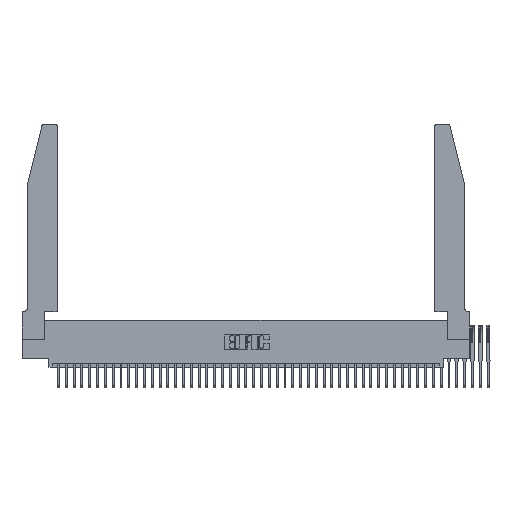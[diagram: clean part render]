
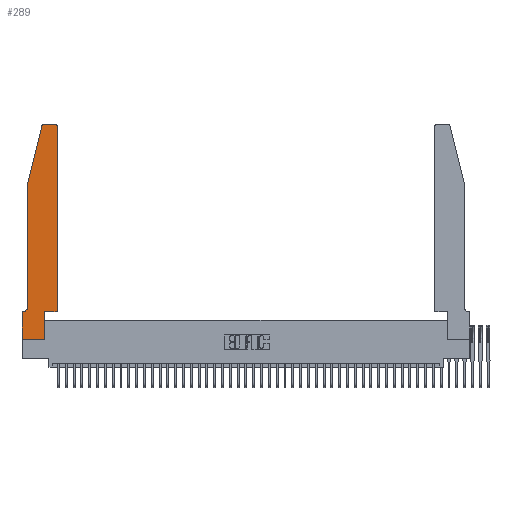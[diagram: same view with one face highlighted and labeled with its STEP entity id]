
A CAD part, top view. The second image highlights one B-rep face of the part: STEP entity #289.
In plain terms, the highlighted planar face has unit normal (0, 0, 1).
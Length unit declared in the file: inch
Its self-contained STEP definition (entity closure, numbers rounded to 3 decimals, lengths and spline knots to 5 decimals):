
#132 = ORIENTED_EDGE ( 'NONE', *, *, #39535, .T. ) ;
#289 = ADVANCED_FACE ( 'NONE', ( #35765 ), #17153, .T. ) ;
#580 = ORIENTED_EDGE ( 'NONE', *, *, #15527, .T. ) ;
#633 = ORIENTED_EDGE ( 'NONE', *, *, #8577, .T. ) ;
#945 = DIRECTION ( 'NONE',  ( 0., 0., 1. ) ) ;
#1299 = CARTESIAN_POINT ( 'NONE',  ( 0.0055, 0.35, 0.37 ) ) ;
#2430 = CIRCLE ( 'NONE', #25621, 0.07 ) ;
#2510 = DIRECTION ( 'NONE',  ( 1., 0., 0. ) ) ;
#2653 = VECTOR ( 'NONE', #2510, 39.37008 ) ;
#2757 = CARTESIAN_POINT ( 'NONE',  ( 0.284, 2.72, 0.37 ) ) ;
#2799 = EDGE_CURVE ( 'NONE', #25915, #9857, #8539, .T. ) ;
#3777 = VERTEX_POINT ( 'NONE', #1299 ) ;
#3970 = DIRECTION ( 'NONE',  ( 0., 1., 0. ) ) ;
#4380 = VECTOR ( 'NONE', #33178, 39.37008 ) ;
#4902 = AXIS2_PLACEMENT_3D ( 'NONE', #39023, #945, #23501 ) ;
#6003 = DIRECTION ( 'NONE',  ( 1., 0., 0. ) ) ;
#6020 = CARTESIAN_POINT ( 'NONE',  ( 0.2865, 0.35, 0.37 ) ) ;
#6171 = CARTESIAN_POINT ( 'NONE',  ( 0., 0., 0.37 ) ) ;
#6260 = VERTEX_POINT ( 'NONE', #23926 ) ;
#6305 = ORIENTED_EDGE ( 'NONE', *, *, #14900, .T. ) ;
#7014 = EDGE_CURVE ( 'NONE', #6260, #27802, #26192, .T. ) ;
#7245 = ORIENTED_EDGE ( 'NONE', *, *, #7014, .T. ) ;
#7323 = CARTESIAN_POINT ( 'NONE',  ( 0.4505, 2.72, 0.37 ) ) ;
#7553 = ORIENTED_EDGE ( 'NONE', *, *, #28223, .T. ) ;
#7808 = VERTEX_POINT ( 'NONE', #19353 ) ;
#8135 = CARTESIAN_POINT ( 'NONE',  ( 0.2865, 0., 0.37 ) ) ;
#8539 = LINE ( 'NONE', #12801, #17133 ) ;
#8577 = EDGE_CURVE ( 'NONE', #31402, #29127, #30892, .T. ) ;
#9243 = VECTOR ( 'NONE', #18280, 39.37008 ) ;
#9857 = VERTEX_POINT ( 'NONE', #14582 ) ;
#10412 = ORIENTED_EDGE ( 'NONE', *, *, #22722, .T. ) ;
#10607 = CARTESIAN_POINT ( 'NONE',  ( 0.4505, 0.35, 0.37 ) ) ;
#11761 = CARTESIAN_POINT ( 'NONE',  ( 0.4205, 2.72, 0.37 ) ) ;
#12193 = DIRECTION ( 'NONE',  ( -1., 0., 0. ) ) ;
#12801 = CARTESIAN_POINT ( 'NONE',  ( 0.0755, 2., 0.37 ) ) ;
#14296 = DIRECTION ( 'NONE',  ( 0., 0., -1. ) ) ;
#14582 = CARTESIAN_POINT ( 'NONE',  ( 0.0755, 0.42, 0.37 ) ) ;
#14900 = EDGE_CURVE ( 'NONE', #24217, #25915, #18774, .T. ) ;
#15026 = DIRECTION ( 'NONE',  ( 1., 0., 0. ) ) ;
#15527 = EDGE_CURVE ( 'NONE', #29127, #24217, #20217, .T. ) ;
#15780 = VECTOR ( 'NONE', #39890, 39.37008 ) ;
#16977 = LINE ( 'NONE', #33323, #34668 ) ;
#17133 = VECTOR ( 'NONE', #34851, 39.37008 ) ;
#17153 = PLANE ( 'NONE',  #4902 ) ;
#17718 = AXIS2_PLACEMENT_3D ( 'NONE', #2757, #25268, #6003 ) ;
#18280 = DIRECTION ( 'NONE',  ( -0.239, -0.971, 0. ) ) ;
#18609 = VERTEX_POINT ( 'NONE', #7323 ) ;
#18774 = LINE ( 'NONE', #33957, #9243 ) ;
#19353 = CARTESIAN_POINT ( 'NONE',  ( 0.4505, 0.35, 0.37 ) ) ;
#19400 = CIRCLE ( 'NONE', #29224, 0.03 ) ;
#19851 = LINE ( 'NONE', #34190, #2653 ) ;
#20217 = CIRCLE ( 'NONE', #17718, 0.03 ) ;
#20818 = DIRECTION ( 'NONE',  ( 1., 0., 0. ) ) ;
#20874 = VECTOR ( 'NONE', #28449, 39.37008 ) ;
#21747 = CARTESIAN_POINT ( 'NONE',  ( 0.25487, 2.72718, 0.37 ) ) ;
#21869 = LINE ( 'NONE', #6020, #20874 ) ;
#22032 = ORIENTED_EDGE ( 'NONE', *, *, #25531, .T. ) ;
#22722 = EDGE_CURVE ( 'NONE', #7808, #18609, #40734, .T. ) ;
#22903 = ORIENTED_EDGE ( 'NONE', *, *, #38307, .T. ) ;
#22919 = VERTEX_POINT ( 'NONE', #8135 ) ;
#23501 = DIRECTION ( 'NONE',  ( 1., 0., 0. ) ) ;
#23926 = CARTESIAN_POINT ( 'NONE',  ( 0., 0.35, 0.37 ) ) ;
#23979 = EDGE_CURVE ( 'NONE', #9857, #3777, #2430, .T. ) ;
#24180 = VECTOR ( 'NONE', #3970, 39.37008 ) ;
#24217 = VERTEX_POINT ( 'NONE', #21747 ) ;
#24406 = CARTESIAN_POINT ( 'NONE',  ( 0., 0., 0.37 ) ) ;
#25268 = DIRECTION ( 'NONE',  ( 0., 0., 1. ) ) ;
#25386 = VERTEX_POINT ( 'NONE', #36580 ) ;
#25531 = EDGE_CURVE ( 'NONE', #3777, #6260, #35341, .T. ) ;
#25621 = AXIS2_PLACEMENT_3D ( 'NONE', #33153, #14296, #36276 ) ;
#25915 = VERTEX_POINT ( 'NONE', #29873 ) ;
#26192 = LINE ( 'NONE', #24406, #15780 ) ;
#27064 = ORIENTED_EDGE ( 'NONE', *, *, #2799, .T. ) ;
#27802 = VERTEX_POINT ( 'NONE', #6171 ) ;
#28018 = CARTESIAN_POINT ( 'NONE',  ( 0.0755, 0.35, 0.37 ) ) ;
#28223 = EDGE_CURVE ( 'NONE', #18609, #31402, #19400, .T. ) ;
#28449 = DIRECTION ( 'NONE',  ( 0., 1., 0. ) ) ;
#29127 = VERTEX_POINT ( 'NONE', #38382 ) ;
#29224 = AXIS2_PLACEMENT_3D ( 'NONE', #11761, #33854, #15026 ) ;
#29873 = CARTESIAN_POINT ( 'NONE',  ( 0.0755, 2., 0.37 ) ) ;
#30892 = LINE ( 'NONE', #36297, #4380 ) ;
#31402 = VERTEX_POINT ( 'NONE', #36600 ) ;
#33153 = CARTESIAN_POINT ( 'NONE',  ( 0.0055, 0.42, 0.37 ) ) ;
#33178 = DIRECTION ( 'NONE',  ( -1., 0., 0. ) ) ;
#33323 = CARTESIAN_POINT ( 'NONE',  ( 0., 0., 0.37 ) ) ;
#33854 = DIRECTION ( 'NONE',  ( 0., 0., 1. ) ) ;
#33957 = CARTESIAN_POINT ( 'NONE',  ( 0.0755, 2., 0.37 ) ) ;
#34029 = ORIENTED_EDGE ( 'NONE', *, *, #23979, .T. ) ;
#34190 = CARTESIAN_POINT ( 'NONE',  ( 0.4505, 0.35, 0.37 ) ) ;
#34368 = VECTOR ( 'NONE', #12193, 39.37008 ) ;
#34668 = VECTOR ( 'NONE', #20818, 39.37008 ) ;
#34851 = DIRECTION ( 'NONE',  ( 0., -1., 0. ) ) ;
#35291 = EDGE_LOOP ( 'NONE', ( #633, #580, #6305, #27064, #34029, #22032, #7245, #39208, #22903, #132, #10412, #7553 ) ) ;
#35341 = LINE ( 'NONE', #28018, #34368 ) ;
#35765 = FACE_OUTER_BOUND ( 'NONE', #35291, .T. ) ;
#36276 = DIRECTION ( 'NONE',  ( -1., 0., 0. ) ) ;
#36297 = CARTESIAN_POINT ( 'NONE',  ( 0.2605, 2.75, 0.37 ) ) ;
#36580 = CARTESIAN_POINT ( 'NONE',  ( 0.2865, 0.35, 0.37 ) ) ;
#36600 = CARTESIAN_POINT ( 'NONE',  ( 0.4205, 2.75, 0.37 ) ) ;
#38307 = EDGE_CURVE ( 'NONE', #22919, #25386, #21869, .T. ) ;
#38382 = CARTESIAN_POINT ( 'NONE',  ( 0.284, 2.75, 0.37 ) ) ;
#38686 = EDGE_CURVE ( 'NONE', #27802, #22919, #16977, .T. ) ;
#39023 = CARTESIAN_POINT ( 'NONE',  ( 0., 0.35, 0.37 ) ) ;
#39208 = ORIENTED_EDGE ( 'NONE', *, *, #38686, .T. ) ;
#39535 = EDGE_CURVE ( 'NONE', #25386, #7808, #19851, .T. ) ;
#39890 = DIRECTION ( 'NONE',  ( 0., -1., 0. ) ) ;
#40734 = LINE ( 'NONE', #10607, #24180 ) ;
